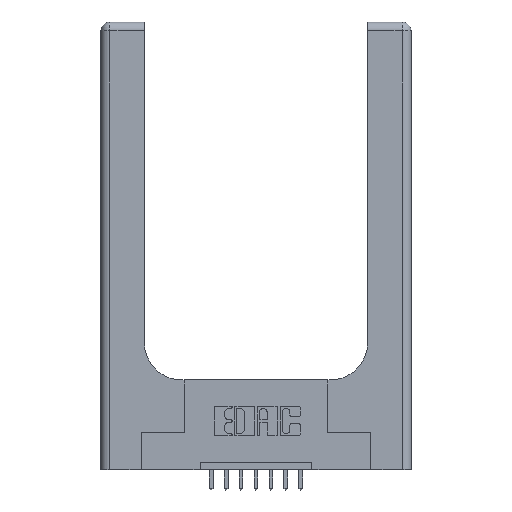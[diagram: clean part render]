
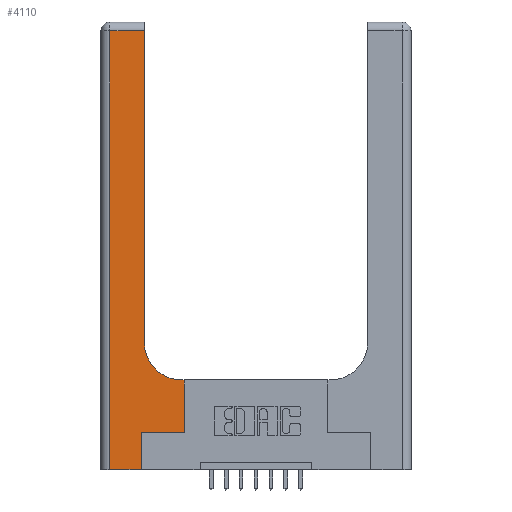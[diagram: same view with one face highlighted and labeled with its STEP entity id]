
A CAD part, top view. The second image highlights one B-rep face of the part: STEP entity #4110.
In plain terms, the highlighted planar face has unit normal (0, 0, 1).
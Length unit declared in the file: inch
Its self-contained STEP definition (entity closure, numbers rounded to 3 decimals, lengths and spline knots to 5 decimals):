
#198 = VECTOR ( 'NONE', #8044, 39.37008 ) ;
#257 = LINE ( 'NONE', #4267, #10674 ) ;
#360 = VECTOR ( 'NONE', #6295, 39.37008 ) ;
#787 = CARTESIAN_POINT ( 'NONE',  ( 0.2915, 0.85, 0.37 ) ) ;
#816 = VECTOR ( 'NONE', #9888, 39.37008 ) ;
#825 = EDGE_CURVE ( 'NONE', #13587, #3722, #2271, .T. ) ;
#990 = VECTOR ( 'NONE', #13862, 39.37008 ) ;
#1043 = DIRECTION ( 'NONE',  ( 1., 0., 0. ) ) ;
#1461 = EDGE_CURVE ( 'NONE', #10464, #13587, #10107, .T. ) ;
#1752 = CARTESIAN_POINT ( 'NONE',  ( 0.5585, 0.25, 0.37 ) ) ;
#1984 = EDGE_CURVE ( 'NONE', #8924, #7401, #7332, .T. ) ;
#2089 = AXIS2_PLACEMENT_3D ( 'NONE', #13476, #14818, #10536 ) ;
#2271 = LINE ( 'NONE', #2344, #8806 ) ;
#2344 = CARTESIAN_POINT ( 'NONE',  ( 0.2915, 0.6, 0.37 ) ) ;
#2809 = EDGE_CURVE ( 'NONE', #8317, #8924, #14346, .T. ) ;
#2999 = VERTEX_POINT ( 'NONE', #5099 ) ;
#3276 = CARTESIAN_POINT ( 'NONE',  ( 0.06, 2.94, 0.37 ) ) ;
#3460 = LINE ( 'NONE', #9801, #360 ) ;
#3722 = VERTEX_POINT ( 'NONE', #11735 ) ;
#3827 = ORIENTED_EDGE ( 'NONE', *, *, #6304, .T. ) ;
#4110 = ADVANCED_FACE ( 'NONE', ( #11726 ), #6388, .F. ) ;
#4232 = VECTOR ( 'NONE', #13812, 39.37008 ) ;
#4267 = CARTESIAN_POINT ( 'NONE',  ( 0., 2.94, 0.37 ) ) ;
#4501 = CARTESIAN_POINT ( 'NONE',  ( 0.06, 3., 0.37 ) ) ;
#5099 = CARTESIAN_POINT ( 'NONE',  ( 0.2915, 2.94, 0.37 ) ) ;
#5297 = VERTEX_POINT ( 'NONE', #787 ) ;
#5375 = EDGE_CURVE ( 'NONE', #5297, #2999, #6227, .T. ) ;
#5725 = CARTESIAN_POINT ( 'NONE',  ( 0.269, 0., 0.37 ) ) ;
#6227 = LINE ( 'NONE', #11497, #198 ) ;
#6295 = DIRECTION ( 'NONE',  ( 1., 0., 0. ) ) ;
#6304 = EDGE_CURVE ( 'NONE', #8035, #10464, #3460, .T. ) ;
#6388 = PLANE ( 'NONE',  #2089 ) ;
#6795 = ORIENTED_EDGE ( 'NONE', *, *, #11852, .T. ) ;
#6804 = CARTESIAN_POINT ( 'NONE',  ( 0.5585, 0.25, 0.37 ) ) ;
#6874 = DIRECTION ( 'NONE',  ( -1., 0., 0. ) ) ;
#7235 = ORIENTED_EDGE ( 'NONE', *, *, #13809, .T. ) ;
#7332 = LINE ( 'NONE', #11645, #4232 ) ;
#7401 = VERTEX_POINT ( 'NONE', #8222 ) ;
#7923 = ORIENTED_EDGE ( 'NONE', *, *, #2809, .T. ) ;
#7997 = DIRECTION ( 'NONE',  ( 0., 0., -1. ) ) ;
#8035 = VERTEX_POINT ( 'NONE', #13589 ) ;
#8044 = DIRECTION ( 'NONE',  ( 0., 1., 0. ) ) ;
#8222 = CARTESIAN_POINT ( 'NONE',  ( 0.269, 0., 0.37 ) ) ;
#8317 = VERTEX_POINT ( 'NONE', #3276 ) ;
#8687 = ORIENTED_EDGE ( 'NONE', *, *, #1984, .T. ) ;
#8806 = VECTOR ( 'NONE', #6874, 39.37008 ) ;
#8924 = VERTEX_POINT ( 'NONE', #9255 ) ;
#9255 = CARTESIAN_POINT ( 'NONE',  ( 0.06, 0., 0.37 ) ) ;
#9801 = CARTESIAN_POINT ( 'NONE',  ( 0.269, 0.25, 0.37 ) ) ;
#9888 = DIRECTION ( 'NONE',  ( 0., 1., 0. ) ) ;
#10107 = LINE ( 'NONE', #1752, #816 ) ;
#10291 = LINE ( 'NONE', #5725, #11397 ) ;
#10464 = VERTEX_POINT ( 'NONE', #6804 ) ;
#10482 = DIRECTION ( 'NONE',  ( 0., 1., 0. ) ) ;
#10536 = DIRECTION ( 'NONE',  ( -1., 0., 0. ) ) ;
#10674 = VECTOR ( 'NONE', #11375, 39.37008 ) ;
#10764 = AXIS2_PLACEMENT_3D ( 'NONE', #15072, #7997, #1043 ) ;
#10865 = CARTESIAN_POINT ( 'NONE',  ( 0.5585, 0.6, 0.37 ) ) ;
#11157 = ORIENTED_EDGE ( 'NONE', *, *, #825, .T. ) ;
#11375 = DIRECTION ( 'NONE',  ( -1., 0., 0. ) ) ;
#11397 = VECTOR ( 'NONE', #10482, 39.37008 ) ;
#11497 = CARTESIAN_POINT ( 'NONE',  ( 0.2915, 3., 0.37 ) ) ;
#11645 = CARTESIAN_POINT ( 'NONE',  ( 0., 0., 0.37 ) ) ;
#11726 = FACE_OUTER_BOUND ( 'NONE', #12101, .T. ) ;
#11735 = CARTESIAN_POINT ( 'NONE',  ( 0.5415, 0.6, 0.37 ) ) ;
#11852 = EDGE_CURVE ( 'NONE', #3722, #5297, #14062, .T. ) ;
#12101 = EDGE_LOOP ( 'NONE', ( #14511, #7235, #7923, #8687, #12870, #3827, #15061, #11157, #6795 ) ) ;
#12870 = ORIENTED_EDGE ( 'NONE', *, *, #14882, .T. ) ;
#13476 = CARTESIAN_POINT ( 'NONE',  ( 0., 3., 0.37 ) ) ;
#13587 = VERTEX_POINT ( 'NONE', #10865 ) ;
#13589 = CARTESIAN_POINT ( 'NONE',  ( 0.269, 0.25, 0.37 ) ) ;
#13809 = EDGE_CURVE ( 'NONE', #2999, #8317, #257, .T. ) ;
#13812 = DIRECTION ( 'NONE',  ( 1., 0., 0. ) ) ;
#13862 = DIRECTION ( 'NONE',  ( 0., -1., 0. ) ) ;
#14062 = CIRCLE ( 'NONE', #10764, 0.25 ) ;
#14346 = LINE ( 'NONE', #4501, #990 ) ;
#14511 = ORIENTED_EDGE ( 'NONE', *, *, #5375, .T. ) ;
#14818 = DIRECTION ( 'NONE',  ( 0., 0., -1. ) ) ;
#14882 = EDGE_CURVE ( 'NONE', #7401, #8035, #10291, .T. ) ;
#15061 = ORIENTED_EDGE ( 'NONE', *, *, #1461, .T. ) ;
#15072 = CARTESIAN_POINT ( 'NONE',  ( 0.5415, 0.85, 0.37 ) ) ;
